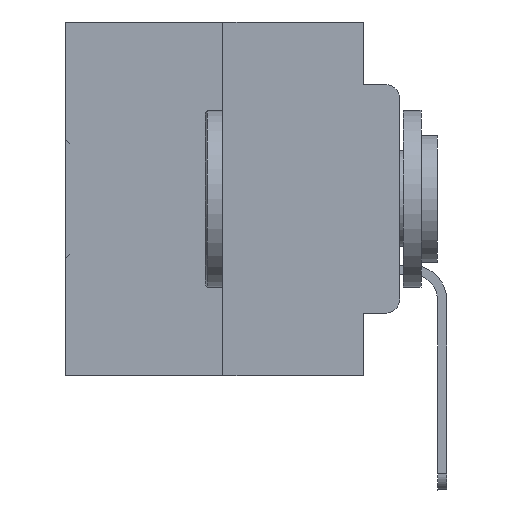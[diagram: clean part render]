
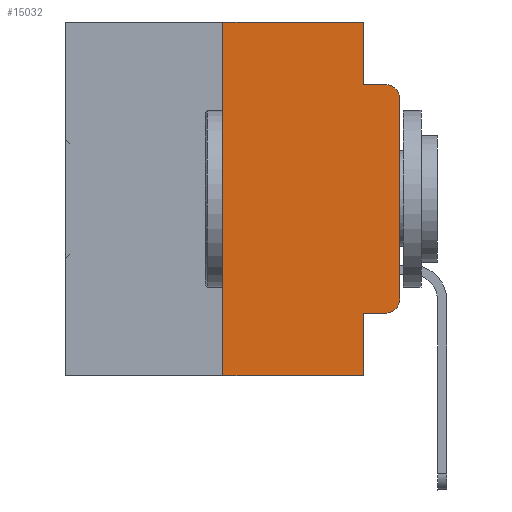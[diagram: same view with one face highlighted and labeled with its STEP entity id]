
A CAD part, left-side view. The second image highlights one B-rep face of the part: STEP entity #15032.
In plain terms, the highlighted planar face has unit normal (-1, 0, 0).
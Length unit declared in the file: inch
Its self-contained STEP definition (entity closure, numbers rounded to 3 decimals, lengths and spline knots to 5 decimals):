
#239 = CARTESIAN_POINT ( 'NONE',  ( 0., 0.051, -0.4115 ) ) ;
#1322 = EDGE_CURVE ( 'NONE', #16744, #21735, #29479, .T. ) ;
#1456 = VERTEX_POINT ( 'NONE', #29328 ) ;
#1779 = VECTOR ( 'NONE', #10435, 39.37008 ) ;
#3009 = CARTESIAN_POINT ( 'NONE',  ( 0., 0., 0. ) ) ;
#3636 = ORIENTED_EDGE ( 'NONE', *, *, #13891, .F. ) ;
#4376 = LINE ( 'NONE', #11485, #27754 ) ;
#5102 = LINE ( 'NONE', #25772, #30994 ) ;
#5318 = DIRECTION ( 'NONE',  ( 0., -1., 0. ) ) ;
#5514 = ORIENTED_EDGE ( 'NONE', *, *, #20449, .T. ) ;
#5755 = VERTEX_POINT ( 'NONE', #11421 ) ;
#6177 = CARTESIAN_POINT ( 'NONE',  ( 0., 0.02, -0.0885 ) ) ;
#7006 = CARTESIAN_POINT ( 'NONE',  ( 0., 0.02, -0.3915 ) ) ;
#7795 = CARTESIAN_POINT ( 'NONE',  ( 0., 0.473, 0. ) ) ;
#8388 = EDGE_LOOP ( 'NONE', ( #5514, #22940, #20967, #10650, #3636, #25479, #28263, #23778, #26320, #13659 ) ) ;
#8414 = LINE ( 'NONE', #3009, #17021 ) ;
#9891 = VECTOR ( 'NONE', #21926, 39.37008 ) ;
#9901 = CARTESIAN_POINT ( 'NONE',  ( 0., 0.051, -0.0885 ) ) ;
#10435 = DIRECTION ( 'NONE',  ( 0., 0., -1. ) ) ;
#10650 = ORIENTED_EDGE ( 'NONE', *, *, #31985, .F. ) ;
#11404 = CARTESIAN_POINT ( 'NONE',  ( 0., 0.051, -0.4115 ) ) ;
#11421 = CARTESIAN_POINT ( 'NONE',  ( 0., 0.051, 0. ) ) ;
#11485 = CARTESIAN_POINT ( 'NONE',  ( 0., 0.473, -0.5 ) ) ;
#12982 = CARTESIAN_POINT ( 'NONE',  ( 0., 0.051, 0. ) ) ;
#13061 = VERTEX_POINT ( 'NONE', #6177 ) ;
#13333 = CARTESIAN_POINT ( 'NONE',  ( 0., 0., -0.3915 ) ) ;
#13529 = CARTESIAN_POINT ( 'NONE',  ( 0., 0.051, 0. ) ) ;
#13659 = ORIENTED_EDGE ( 'NONE', *, *, #1322, .T. ) ;
#13891 = EDGE_CURVE ( 'NONE', #16623, #5755, #5102, .T. ) ;
#14147 = EDGE_CURVE ( 'NONE', #1456, #25196, #4376, .T. ) ;
#14383 = EDGE_CURVE ( 'NONE', #17335, #16744, #16660, .T. ) ;
#15032 = ADVANCED_FACE ( 'NONE', ( #31044 ), #25436, .F. ) ;
#15152 = CARTESIAN_POINT ( 'NONE',  ( 0., 0.051, -0.0885 ) ) ;
#15289 = CARTESIAN_POINT ( 'NONE',  ( 0., 0.25, 0. ) ) ;
#16264 = CARTESIAN_POINT ( 'NONE',  ( 0., 0.25, 0. ) ) ;
#16623 = VERTEX_POINT ( 'NONE', #16264 ) ;
#16660 = LINE ( 'NONE', #11404, #9891 ) ;
#16744 = VERTEX_POINT ( 'NONE', #27091 ) ;
#17021 = VECTOR ( 'NONE', #21294, 39.37008 ) ;
#17334 = DIRECTION ( 'NONE',  ( -1., 0., 0. ) ) ;
#17335 = VERTEX_POINT ( 'NONE', #239 ) ;
#18476 = VECTOR ( 'NONE', #5318, 39.37008 ) ;
#18523 = EDGE_CURVE ( 'NONE', #22974, #13061, #27772, .T. ) ;
#20178 = DIRECTION ( 'NONE',  ( 1., 0., 0. ) ) ;
#20449 = EDGE_CURVE ( 'NONE', #21735, #22974, #8414, .T. ) ;
#20544 = DIRECTION ( 'NONE',  ( 0., 0., 1. ) ) ;
#20967 = ORIENTED_EDGE ( 'NONE', *, *, #24352, .F. ) ;
#21294 = DIRECTION ( 'NONE',  ( 0., 0., 1. ) ) ;
#21735 = VERTEX_POINT ( 'NONE', #13333 ) ;
#21926 = DIRECTION ( 'NONE',  ( 0., -1., 0. ) ) ;
#22318 = DIRECTION ( 'NONE',  ( -1., 0., 0. ) ) ;
#22340 = DIRECTION ( 'NONE',  ( 0., -1., 0. ) ) ;
#22609 = DIRECTION ( 'NONE',  ( 0., 0., -1. ) ) ;
#22940 = ORIENTED_EDGE ( 'NONE', *, *, #18523, .T. ) ;
#22974 = VERTEX_POINT ( 'NONE', #23339 ) ;
#23230 = DIRECTION ( 'NONE',  ( 0., 0., -1. ) ) ;
#23339 = CARTESIAN_POINT ( 'NONE',  ( 0., 0., -0.1085 ) ) ;
#23376 = AXIS2_PLACEMENT_3D ( 'NONE', #7795, #20178, #23230 ) ;
#23778 = ORIENTED_EDGE ( 'NONE', *, *, #25292, .F. ) ;
#23868 = LINE ( 'NONE', #13529, #30188 ) ;
#24352 = EDGE_CURVE ( 'NONE', #31082, #13061, #30929, .T. ) ;
#24501 = AXIS2_PLACEMENT_3D ( 'NONE', #29958, #22318, #32678 ) ;
#25196 = VERTEX_POINT ( 'NONE', #32053 ) ;
#25292 = EDGE_CURVE ( 'NONE', #17335, #25196, #25709, .T. ) ;
#25436 = PLANE ( 'NONE',  #23376 ) ;
#25479 = ORIENTED_EDGE ( 'NONE', *, *, #33524, .F. ) ;
#25635 = LINE ( 'NONE', #15289, #30263 ) ;
#25709 = LINE ( 'NONE', #12982, #1779 ) ;
#25772 = CARTESIAN_POINT ( 'NONE',  ( 0., 0.473, 0. ) ) ;
#26320 = ORIENTED_EDGE ( 'NONE', *, *, #14383, .T. ) ;
#27091 = CARTESIAN_POINT ( 'NONE',  ( 0., 0.02, -0.4115 ) ) ;
#27754 = VECTOR ( 'NONE', #22340, 39.37008 ) ;
#27772 = CIRCLE ( 'NONE', #24501, 0.02 ) ;
#28263 = ORIENTED_EDGE ( 'NONE', *, *, #14147, .T. ) ;
#28383 = AXIS2_PLACEMENT_3D ( 'NONE', #7006, #17334, #22609 ) ;
#29294 = DIRECTION ( 'NONE',  ( 0., 0., -1. ) ) ;
#29328 = CARTESIAN_POINT ( 'NONE',  ( 0., 0.25, -0.5 ) ) ;
#29479 = CIRCLE ( 'NONE', #28383, 0.02 ) ;
#29958 = CARTESIAN_POINT ( 'NONE',  ( 0., 0.02, -0.1085 ) ) ;
#30188 = VECTOR ( 'NONE', #29294, 39.37008 ) ;
#30263 = VECTOR ( 'NONE', #20544, 39.37008 ) ;
#30929 = LINE ( 'NONE', #15152, #18476 ) ;
#30994 = VECTOR ( 'NONE', #31037, 39.37008 ) ;
#31037 = DIRECTION ( 'NONE',  ( 0., -1., 0. ) ) ;
#31044 = FACE_OUTER_BOUND ( 'NONE', #8388, .T. ) ;
#31082 = VERTEX_POINT ( 'NONE', #9901 ) ;
#31985 = EDGE_CURVE ( 'NONE', #5755, #31082, #23868, .T. ) ;
#32053 = CARTESIAN_POINT ( 'NONE',  ( 0., 0.051, -0.5 ) ) ;
#32678 = DIRECTION ( 'NONE',  ( 0., 0., -1. ) ) ;
#33524 = EDGE_CURVE ( 'NONE', #1456, #16623, #25635, .T. ) ;
